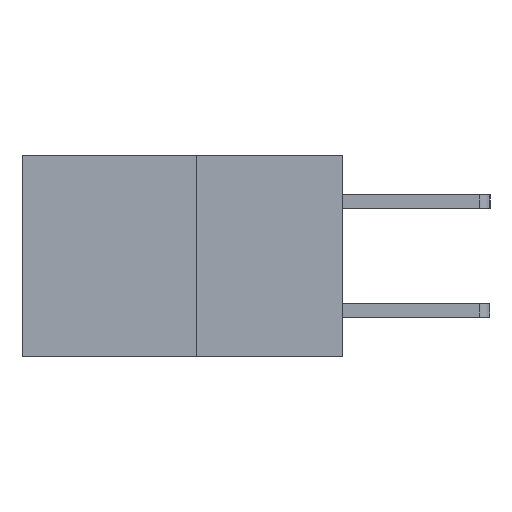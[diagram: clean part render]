
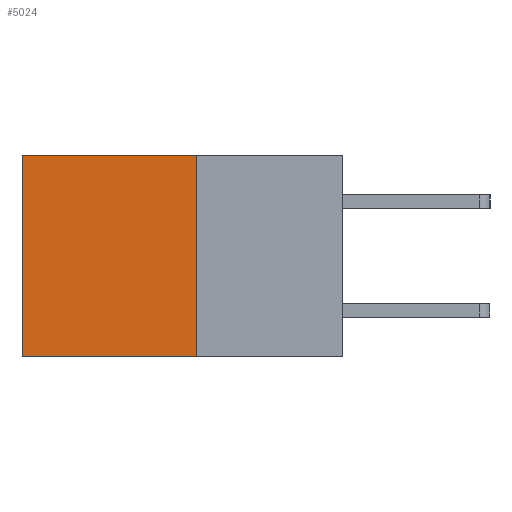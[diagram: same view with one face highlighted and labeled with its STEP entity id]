
A CAD part, left-side view. The second image highlights one B-rep face of the part: STEP entity #5024.
In plain terms, the highlighted planar face has unit normal (-1, 0, 0).
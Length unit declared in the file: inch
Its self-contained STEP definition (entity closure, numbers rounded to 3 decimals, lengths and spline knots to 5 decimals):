
#426 = LINE ( 'NONE', #3939, #4025 ) ;
#861 = CARTESIAN_POINT ( 'NONE',  ( 0.277, 0.27, -0.37 ) ) ;
#1547 = VECTOR ( 'NONE', #2767, 39.37008 ) ;
#1723 = AXIS2_PLACEMENT_3D ( 'NONE', #8756, #5764, #4253 ) ;
#1775 = VECTOR ( 'NONE', #3803, 39.37008 ) ;
#1791 = CARTESIAN_POINT ( 'NONE',  ( 0.277, 0.59, 0. ) ) ;
#1961 = LINE ( 'NONE', #4588, #5842 ) ;
#2149 = VERTEX_POINT ( 'NONE', #861 ) ;
#2767 = DIRECTION ( 'NONE',  ( 0., 0., -1. ) ) ;
#2928 = EDGE_CURVE ( 'NONE', #8422, #7813, #1961, .T. ) ;
#3119 = CARTESIAN_POINT ( 'NONE',  ( 0.277, 0.59, -0.37 ) ) ;
#3217 = EDGE_LOOP ( 'NONE', ( #9398, #8476, #9705, #9578 ) ) ;
#3563 = LINE ( 'NONE', #3119, #1547 ) ;
#3676 = DIRECTION ( 'NONE',  ( 0., 0., -1. ) ) ;
#3803 = DIRECTION ( 'NONE',  ( 0., 1., 0. ) ) ;
#3892 = CARTESIAN_POINT ( 'NONE',  ( 0.277, 0.27, -0.37 ) ) ;
#3939 = CARTESIAN_POINT ( 'NONE',  ( 0.277, 0.27, -0.37 ) ) ;
#4025 = VECTOR ( 'NONE', #3676, 39.37008 ) ;
#4071 = EDGE_CURVE ( 'NONE', #2149, #8438, #7690, .T. ) ;
#4253 = DIRECTION ( 'NONE',  ( 0., 0., -1. ) ) ;
#4588 = CARTESIAN_POINT ( 'NONE',  ( 0.277, 0.27, 0. ) ) ;
#5024 = ADVANCED_FACE ( 'NONE', ( #9844 ), #7599, .F. ) ;
#5719 = CARTESIAN_POINT ( 'NONE',  ( 0.277, 0.59, -0.37 ) ) ;
#5764 = DIRECTION ( 'NONE',  ( 1., 0., 0. ) ) ;
#5803 = CARTESIAN_POINT ( 'NONE',  ( 0.277, 0.27, 0. ) ) ;
#5842 = VECTOR ( 'NONE', #9714, 39.37008 ) ;
#7599 = PLANE ( 'NONE',  #1723 ) ;
#7690 = LINE ( 'NONE', #3892, #1775 ) ;
#7813 = VERTEX_POINT ( 'NONE', #1791 ) ;
#8422 = VERTEX_POINT ( 'NONE', #5803 ) ;
#8438 = VERTEX_POINT ( 'NONE', #5719 ) ;
#8476 = ORIENTED_EDGE ( 'NONE', *, *, #4071, .F. ) ;
#8756 = CARTESIAN_POINT ( 'NONE',  ( 0.277, 0.27, -0.37 ) ) ;
#8835 = EDGE_CURVE ( 'NONE', #7813, #8438, #3563, .T. ) ;
#9383 = EDGE_CURVE ( 'NONE', #8422, #2149, #426, .T. ) ;
#9398 = ORIENTED_EDGE ( 'NONE', *, *, #8835, .T. ) ;
#9578 = ORIENTED_EDGE ( 'NONE', *, *, #2928, .T. ) ;
#9705 = ORIENTED_EDGE ( 'NONE', *, *, #9383, .F. ) ;
#9714 = DIRECTION ( 'NONE',  ( 0., 1., 0. ) ) ;
#9844 = FACE_OUTER_BOUND ( 'NONE', #3217, .T. ) ;
